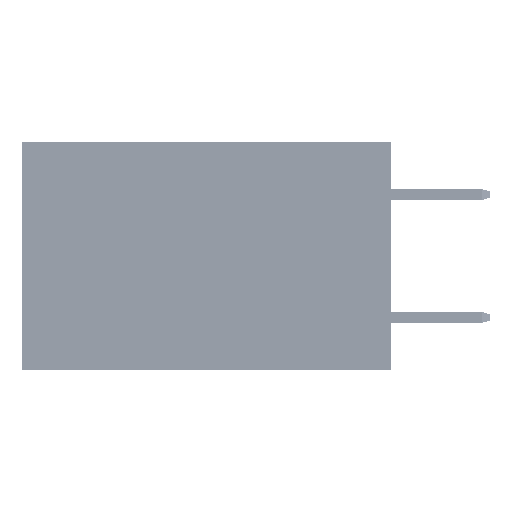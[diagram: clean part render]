
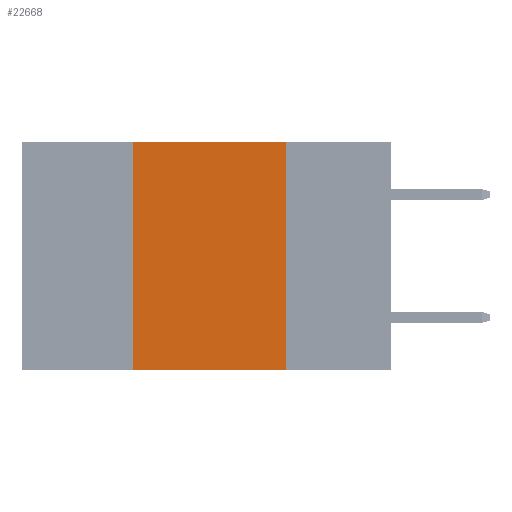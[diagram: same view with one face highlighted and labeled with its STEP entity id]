
A CAD part, left-side view. The second image highlights one B-rep face of the part: STEP entity #22668.
In plain terms, the highlighted planar face has unit normal (-1, 0, 0).
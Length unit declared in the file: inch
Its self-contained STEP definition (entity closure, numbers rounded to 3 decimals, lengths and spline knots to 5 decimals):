
#4945 = LINE ( 'NONE', #19565, #35356 ) ;
#5836 = VECTOR ( 'NONE', #10179, 39.37008 ) ;
#10179 = DIRECTION ( 'NONE',  ( 0., 0., -1. ) ) ;
#10464 = EDGE_CURVE ( 'NONE', #48093, #34240, #20777, .T. ) ;
#11927 = CARTESIAN_POINT ( 'NONE',  ( 0., 0.42, -0.37 ) ) ;
#12153 = PLANE ( 'NONE',  #36906 ) ;
#12361 = DIRECTION ( 'NONE',  ( 0., 0., 1. ) ) ;
#13166 = EDGE_CURVE ( 'NONE', #15588, #37826, #4945, .T. ) ;
#15588 = VERTEX_POINT ( 'NONE', #11927 ) ;
#16332 = DIRECTION ( 'NONE',  ( 0., 0., -1. ) ) ;
#16562 = FACE_OUTER_BOUND ( 'NONE', #28138, .T. ) ;
#19565 = CARTESIAN_POINT ( 'NONE',  ( 0., 0.42, 0. ) ) ;
#20330 = EDGE_CURVE ( 'NONE', #37826, #48093, #27336, .T. ) ;
#20777 = LINE ( 'NONE', #37053, #5836 ) ;
#20864 = ORIENTED_EDGE ( 'NONE', *, *, #10464, .F. ) ;
#22181 = CARTESIAN_POINT ( 'NONE',  ( 0., 0.6, 0. ) ) ;
#22668 = ADVANCED_FACE ( 'NONE', ( #16562 ), #12153, .F. ) ;
#23462 = CARTESIAN_POINT ( 'NONE',  ( 0., 0.42, 0. ) ) ;
#24395 = CARTESIAN_POINT ( 'NONE',  ( 0., 0.17, -0.37 ) ) ;
#26044 = DIRECTION ( 'NONE',  ( 0., -1., 0. ) ) ;
#27336 = LINE ( 'NONE', #22181, #28530 ) ;
#28138 = EDGE_LOOP ( 'NONE', ( #20864, #36403, #38231, #47727 ) ) ;
#28530 = VECTOR ( 'NONE', #33335, 39.37008 ) ;
#29529 = CARTESIAN_POINT ( 'NONE',  ( 0., 0.6, -0.37 ) ) ;
#31172 = CARTESIAN_POINT ( 'NONE',  ( 0., 0.6, 0. ) ) ;
#33335 = DIRECTION ( 'NONE',  ( 0., -1., 0. ) ) ;
#34240 = VERTEX_POINT ( 'NONE', #24395 ) ;
#34870 = LINE ( 'NONE', #29529, #48533 ) ;
#35356 = VECTOR ( 'NONE', #12361, 39.37008 ) ;
#35363 = CARTESIAN_POINT ( 'NONE',  ( 0., 0.17, 0. ) ) ;
#36403 = ORIENTED_EDGE ( 'NONE', *, *, #20330, .F. ) ;
#36906 = AXIS2_PLACEMENT_3D ( 'NONE', #31172, #39009, #16332 ) ;
#37053 = CARTESIAN_POINT ( 'NONE',  ( 0., 0.17, 0. ) ) ;
#37826 = VERTEX_POINT ( 'NONE', #23462 ) ;
#38231 = ORIENTED_EDGE ( 'NONE', *, *, #13166, .F. ) ;
#39009 = DIRECTION ( 'NONE',  ( 1., 0., 0. ) ) ;
#47727 = ORIENTED_EDGE ( 'NONE', *, *, #47921, .T. ) ;
#47921 = EDGE_CURVE ( 'NONE', #15588, #34240, #34870, .T. ) ;
#48093 = VERTEX_POINT ( 'NONE', #35363 ) ;
#48533 = VECTOR ( 'NONE', #26044, 39.37008 ) ;
